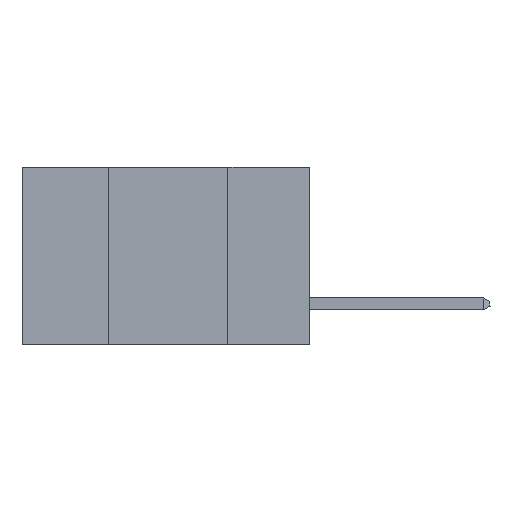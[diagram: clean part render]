
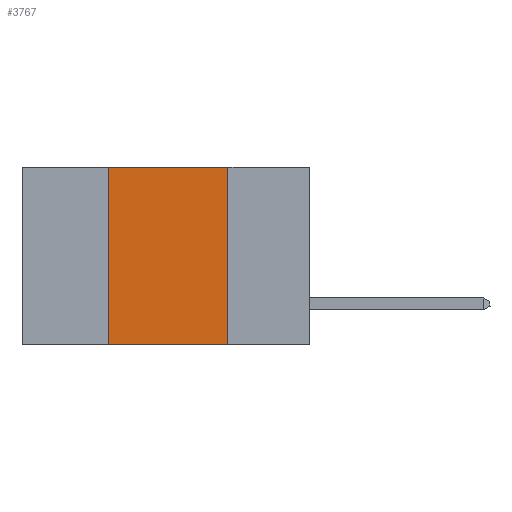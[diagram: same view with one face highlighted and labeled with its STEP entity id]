
A CAD part, left-side view. The second image highlights one B-rep face of the part: STEP entity #3767.
In plain terms, the highlighted planar face has unit normal (-1, 0, 0).
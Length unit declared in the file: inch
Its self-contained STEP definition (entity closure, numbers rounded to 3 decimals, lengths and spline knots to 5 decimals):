
#247 = CARTESIAN_POINT ( 'NONE',  ( 0., 0.6, 0. ) ) ;
#1372 = ORIENTED_EDGE ( 'NONE', *, *, #12594, .F. ) ;
#2327 = LINE ( 'NONE', #21583, #14011 ) ;
#3225 = VECTOR ( 'NONE', #8937, 39.37008 ) ;
#3328 = CARTESIAN_POINT ( 'NONE',  ( 0., 0.42, 0. ) ) ;
#3767 = ADVANCED_FACE ( 'NONE', ( #4020 ), #21886, .F. ) ;
#4020 = FACE_OUTER_BOUND ( 'NONE', #17106, .T. ) ;
#5512 = DIRECTION ( 'NONE',  ( 0., 0., 1. ) ) ;
#8937 = DIRECTION ( 'NONE',  ( 0., -1., 0. ) ) ;
#9169 = EDGE_CURVE ( 'NONE', #24904, #22318, #17565, .T. ) ;
#9729 = AXIS2_PLACEMENT_3D ( 'NONE', #20108, #15328, #11624 ) ;
#10971 = CARTESIAN_POINT ( 'NONE',  ( 0., 0.17, -0.37 ) ) ;
#11371 = ORIENTED_EDGE ( 'NONE', *, *, #9169, .T. ) ;
#11624 = DIRECTION ( 'NONE',  ( 0., 0., -1. ) ) ;
#12356 = VERTEX_POINT ( 'NONE', #21019 ) ;
#12520 = EDGE_CURVE ( 'NONE', #24904, #28169, #27159, .T. ) ;
#12594 = EDGE_CURVE ( 'NONE', #12356, #22318, #2327, .T. ) ;
#14011 = VECTOR ( 'NONE', #19525, 39.37008 ) ;
#14283 = CARTESIAN_POINT ( 'NONE',  ( 0., 0.42, 0. ) ) ;
#14459 = DIRECTION ( 'NONE',  ( 0., -1., 0. ) ) ;
#15281 = LINE ( 'NONE', #247, #3225 ) ;
#15328 = DIRECTION ( 'NONE',  ( 1., 0., 0. ) ) ;
#15633 = EDGE_CURVE ( 'NONE', #28169, #12356, #15281, .T. ) ;
#15934 = ORIENTED_EDGE ( 'NONE', *, *, #15633, .F. ) ;
#17106 = EDGE_LOOP ( 'NONE', ( #1372, #15934, #23165, #11371 ) ) ;
#17565 = LINE ( 'NONE', #23559, #28526 ) ;
#19525 = DIRECTION ( 'NONE',  ( 0., 0., -1. ) ) ;
#20108 = CARTESIAN_POINT ( 'NONE',  ( 0., 0.6, 0. ) ) ;
#21019 = CARTESIAN_POINT ( 'NONE',  ( 0., 0.17, 0. ) ) ;
#21127 = VECTOR ( 'NONE', #5512, 39.37008 ) ;
#21583 = CARTESIAN_POINT ( 'NONE',  ( 0., 0.17, 0. ) ) ;
#21886 = PLANE ( 'NONE',  #9729 ) ;
#22318 = VERTEX_POINT ( 'NONE', #10971 ) ;
#22327 = CARTESIAN_POINT ( 'NONE',  ( 0., 0.42, -0.37 ) ) ;
#23165 = ORIENTED_EDGE ( 'NONE', *, *, #12520, .F. ) ;
#23559 = CARTESIAN_POINT ( 'NONE',  ( 0., 0.6, -0.37 ) ) ;
#24904 = VERTEX_POINT ( 'NONE', #22327 ) ;
#27159 = LINE ( 'NONE', #3328, #21127 ) ;
#28169 = VERTEX_POINT ( 'NONE', #14283 ) ;
#28526 = VECTOR ( 'NONE', #14459, 39.37008 ) ;
